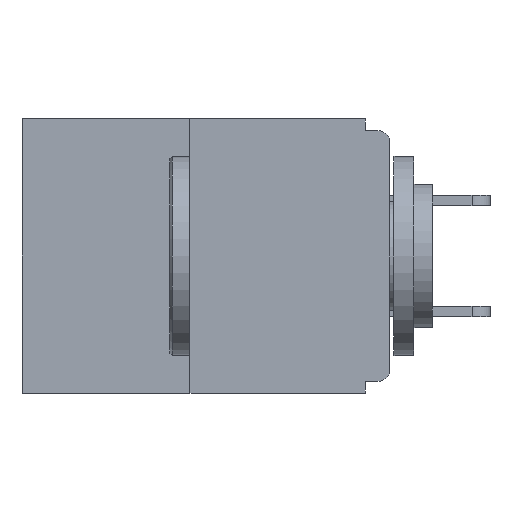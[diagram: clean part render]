
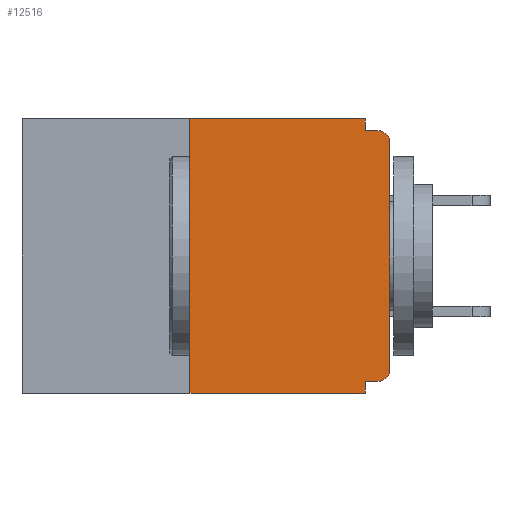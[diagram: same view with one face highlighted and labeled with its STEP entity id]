
A CAD part, left-side view. The second image highlights one B-rep face of the part: STEP entity #12516.
In plain terms, the highlighted planar face has unit normal (-1, 0, 0).
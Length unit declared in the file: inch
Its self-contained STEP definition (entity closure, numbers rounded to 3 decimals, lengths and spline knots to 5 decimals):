
#1549 = DIRECTION ( 'NONE',  ( 0., 0., -1. ) ) ;
#1602 = AXIS2_PLACEMENT_3D ( 'NONE', #13497, #18033, #15996 ) ;
#2982 = DIRECTION ( 'NONE',  ( 0., 0., -1. ) ) ;
#3003 = VERTEX_POINT ( 'NONE', #20035 ) ;
#3995 = ORIENTED_EDGE ( 'NONE', *, *, #11751, .T. ) ;
#4500 = CIRCLE ( 'NONE', #6083, 0.015 ) ;
#4677 = VECTOR ( 'NONE', #5115, 39.37008 ) ;
#4814 = VERTEX_POINT ( 'NONE', #20012 ) ;
#5018 = CARTESIAN_POINT ( 'NONE',  ( 0., 0.031, 0. ) ) ;
#5079 = EDGE_CURVE ( 'NONE', #3003, #9491, #16593, .T. ) ;
#5115 = DIRECTION ( 'NONE',  ( 0., 0., -1. ) ) ;
#5555 = VERTEX_POINT ( 'NONE', #29934 ) ;
#5968 = ORIENTED_EDGE ( 'NONE', *, *, #24614, .F. ) ;
#6083 = AXIS2_PLACEMENT_3D ( 'NONE', #17814, #6493, #1549 ) ;
#6114 = DIRECTION ( 'NONE',  ( 0., -1., 0. ) ) ;
#6493 = DIRECTION ( 'NONE',  ( -1., 0., 0. ) ) ;
#6513 = CARTESIAN_POINT ( 'NONE',  ( 0., 0., -0.328 ) ) ;
#6549 = VERTEX_POINT ( 'NONE', #18488 ) ;
#7219 = EDGE_LOOP ( 'NONE', ( #21974, #13508, #12035, #19053, #17296, #3995, #19390, #24775, #5968, #26868 ) ) ;
#7614 = LINE ( 'NONE', #15676, #22498 ) ;
#7864 = VECTOR ( 'NONE', #9344, 39.37008 ) ;
#8834 = DIRECTION ( 'NONE',  ( 0., 1., 0. ) ) ;
#9085 = CARTESIAN_POINT ( 'NONE',  ( 0., 0.031, -0.015 ) ) ;
#9344 = DIRECTION ( 'NONE',  ( 0., -1., 0. ) ) ;
#9418 = VECTOR ( 'NONE', #8834, 39.37008 ) ;
#9491 = VERTEX_POINT ( 'NONE', #9085 ) ;
#9958 = CARTESIAN_POINT ( 'NONE',  ( 0., 0., 0. ) ) ;
#10157 = LINE ( 'NONE', #6513, #9418 ) ;
#11138 = CARTESIAN_POINT ( 'NONE',  ( 0., 0.015, -0.015 ) ) ;
#11401 = EDGE_CURVE ( 'NONE', #29859, #5555, #29480, .T. ) ;
#11751 = EDGE_CURVE ( 'NONE', #6549, #4814, #29452, .T. ) ;
#11812 = CARTESIAN_POINT ( 'NONE',  ( 0., 0.015, -0.313 ) ) ;
#12035 = ORIENTED_EDGE ( 'NONE', *, *, #17872, .T. ) ;
#12186 = LINE ( 'NONE', #29439, #20897 ) ;
#12516 = ADVANCED_FACE ( 'NONE', ( #29417 ), #18133, .F. ) ;
#12565 = EDGE_CURVE ( 'NONE', #6549, #29859, #10157, .T. ) ;
#12964 = CARTESIAN_POINT ( 'NONE',  ( 0., 0.031, -0.328 ) ) ;
#13209 = AXIS2_PLACEMENT_3D ( 'NONE', #11812, #16442, #16646 ) ;
#13497 = CARTESIAN_POINT ( 'NONE',  ( 0., 0.46, 0. ) ) ;
#13508 = ORIENTED_EDGE ( 'NONE', *, *, #23027, .F. ) ;
#13664 = EDGE_CURVE ( 'NONE', #26928, #24733, #4500, .T. ) ;
#14491 = VECTOR ( 'NONE', #21788, 39.37008 ) ;
#15676 = CARTESIAN_POINT ( 'NONE',  ( 0., 0., -0.015 ) ) ;
#15996 = DIRECTION ( 'NONE',  ( 0., 0., -1. ) ) ;
#16442 = DIRECTION ( 'NONE',  ( -1., 0., 0. ) ) ;
#16593 = LINE ( 'NONE', #5018, #4677 ) ;
#16646 = DIRECTION ( 'NONE',  ( 0., 0., -1. ) ) ;
#17296 = ORIENTED_EDGE ( 'NONE', *, *, #12565, .F. ) ;
#17814 = CARTESIAN_POINT ( 'NONE',  ( 0., 0.015, -0.03 ) ) ;
#17872 = EDGE_CURVE ( 'NONE', #23101, #5555, #26758, .T. ) ;
#18033 = DIRECTION ( 'NONE',  ( 1., 0., 0. ) ) ;
#18133 = PLANE ( 'NONE',  #1602 ) ;
#18187 = EDGE_CURVE ( 'NONE', #20799, #3003, #12186, .T. ) ;
#18488 = CARTESIAN_POINT ( 'NONE',  ( 0., 0.015, -0.328 ) ) ;
#19053 = ORIENTED_EDGE ( 'NONE', *, *, #11401, .F. ) ;
#19366 = DIRECTION ( 'NONE',  ( 0., 0., 1. ) ) ;
#19390 = ORIENTED_EDGE ( 'NONE', *, *, #28671, .T. ) ;
#19638 = CARTESIAN_POINT ( 'NONE',  ( 0., 0.25, 0. ) ) ;
#19861 = CARTESIAN_POINT ( 'NONE',  ( 0., 0., -0.03 ) ) ;
#20012 = CARTESIAN_POINT ( 'NONE',  ( 0., 0., -0.313 ) ) ;
#20035 = CARTESIAN_POINT ( 'NONE',  ( 0., 0.031, 0. ) ) ;
#20799 = VERTEX_POINT ( 'NONE', #25712 ) ;
#20897 = VECTOR ( 'NONE', #6114, 39.37008 ) ;
#20946 = CARTESIAN_POINT ( 'NONE',  ( 0., 0.25, -0.343 ) ) ;
#21788 = DIRECTION ( 'NONE',  ( 0., 0., 1. ) ) ;
#21974 = ORIENTED_EDGE ( 'NONE', *, *, #18187, .F. ) ;
#22498 = VECTOR ( 'NONE', #29413, 39.37008 ) ;
#23027 = EDGE_CURVE ( 'NONE', #23101, #20799, #25787, .T. ) ;
#23101 = VERTEX_POINT ( 'NONE', #20946 ) ;
#23270 = VECTOR ( 'NONE', #2982, 39.37008 ) ;
#23649 = CARTESIAN_POINT ( 'NONE',  ( 0., 0.031, -0.343 ) ) ;
#24614 = EDGE_CURVE ( 'NONE', #9491, #24733, #7614, .T. ) ;
#24733 = VERTEX_POINT ( 'NONE', #11138 ) ;
#24775 = ORIENTED_EDGE ( 'NONE', *, *, #13664, .T. ) ;
#25712 = CARTESIAN_POINT ( 'NONE',  ( 0., 0.25, 0. ) ) ;
#25787 = LINE ( 'NONE', #19638, #14491 ) ;
#26076 = VECTOR ( 'NONE', #19366, 39.37008 ) ;
#26758 = LINE ( 'NONE', #27620, #7864 ) ;
#26868 = ORIENTED_EDGE ( 'NONE', *, *, #5079, .F. ) ;
#26928 = VERTEX_POINT ( 'NONE', #19861 ) ;
#27620 = CARTESIAN_POINT ( 'NONE',  ( 0., 0.46, -0.343 ) ) ;
#27868 = LINE ( 'NONE', #9958, #26076 ) ;
#28671 = EDGE_CURVE ( 'NONE', #4814, #26928, #27868, .T. ) ;
#29413 = DIRECTION ( 'NONE',  ( 0., -1., 0. ) ) ;
#29417 = FACE_OUTER_BOUND ( 'NONE', #7219, .T. ) ;
#29439 = CARTESIAN_POINT ( 'NONE',  ( 0., 0.46, 0. ) ) ;
#29452 = CIRCLE ( 'NONE', #13209, 0.015 ) ;
#29480 = LINE ( 'NONE', #23649, #23270 ) ;
#29859 = VERTEX_POINT ( 'NONE', #12964 ) ;
#29934 = CARTESIAN_POINT ( 'NONE',  ( 0., 0.031, -0.343 ) ) ;
